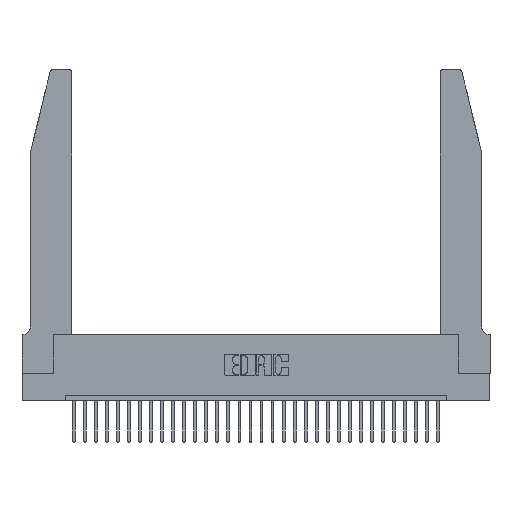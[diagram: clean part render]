
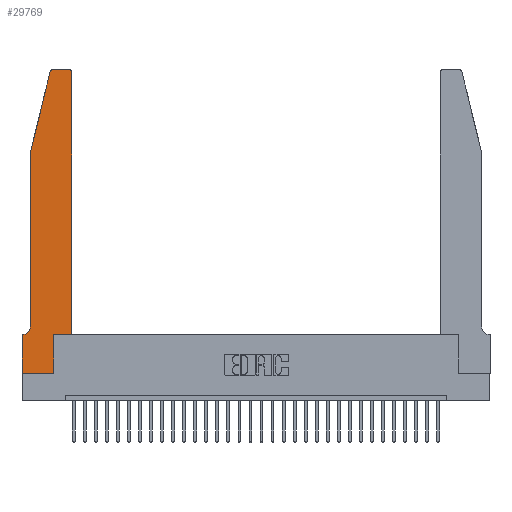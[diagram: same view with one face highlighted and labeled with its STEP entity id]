
A CAD part, top view. The second image highlights one B-rep face of the part: STEP entity #29769.
In plain terms, the highlighted planar face has unit normal (0, 0, 1).
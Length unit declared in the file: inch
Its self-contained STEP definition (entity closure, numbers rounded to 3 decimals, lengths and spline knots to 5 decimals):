
#386 = ORIENTED_EDGE ( 'NONE', *, *, #17840, .T. ) ;
#1127 = LINE ( 'NONE', #2753, #26141 ) ;
#1142 = EDGE_CURVE ( 'NONE', #30570, #8657, #6463, .T. ) ;
#1727 = ORIENTED_EDGE ( 'NONE', *, *, #22648, .T. ) ;
#2080 = ORIENTED_EDGE ( 'NONE', *, *, #17526, .T. ) ;
#2753 = CARTESIAN_POINT ( 'NONE',  ( 0., 0., 0.37 ) ) ;
#3370 = VECTOR ( 'NONE', #25159, 39.37008 ) ;
#3501 = EDGE_CURVE ( 'NONE', #26443, #23081, #20427, .T. ) ;
#3567 = CARTESIAN_POINT ( 'NONE',  ( 0.25487, 2.72718, 0.37 ) ) ;
#3782 = ORIENTED_EDGE ( 'NONE', *, *, #3501, .T. ) ;
#3824 = ORIENTED_EDGE ( 'NONE', *, *, #29797, .T. ) ;
#4398 = VERTEX_POINT ( 'NONE', #22264 ) ;
#4504 = VERTEX_POINT ( 'NONE', #17373 ) ;
#4585 = CARTESIAN_POINT ( 'NONE',  ( 0.284, 2.75, 0.37 ) ) ;
#4661 = DIRECTION ( 'NONE',  ( -1., 0., 0. ) ) ;
#4742 = VERTEX_POINT ( 'NONE', #24106 ) ;
#5469 = CARTESIAN_POINT ( 'NONE',  ( 0.0055, 0.42, 0.37 ) ) ;
#5599 = CARTESIAN_POINT ( 'NONE',  ( 0.4205, 2.72, 0.37 ) ) ;
#5793 = EDGE_CURVE ( 'NONE', #19160, #30570, #7446, .T. ) ;
#5992 = EDGE_CURVE ( 'NONE', #17692, #19160, #17774, .T. ) ;
#6463 = LINE ( 'NONE', #16593, #26981 ) ;
#6670 = CARTESIAN_POINT ( 'NONE',  ( 0.2865, 0.35, 0.37 ) ) ;
#6869 = CARTESIAN_POINT ( 'NONE',  ( 0.0755, 0.42, 0.37 ) ) ;
#7446 = LINE ( 'NONE', #19757, #18492 ) ;
#8516 = LINE ( 'NONE', #20334, #27184 ) ;
#8657 = VERTEX_POINT ( 'NONE', #20517 ) ;
#8892 = AXIS2_PLACEMENT_3D ( 'NONE', #27318, #10089, #29645 ) ;
#10089 = DIRECTION ( 'NONE',  ( 0., 0., 1. ) ) ;
#10143 = CARTESIAN_POINT ( 'NONE',  ( 0.2865, 0., 0.37 ) ) ;
#10771 = CARTESIAN_POINT ( 'NONE',  ( 0.0755, 2., 0.37 ) ) ;
#11291 = AXIS2_PLACEMENT_3D ( 'NONE', #27268, #14144, #31194 ) ;
#11407 = ORIENTED_EDGE ( 'NONE', *, *, #29382, .T. ) ;
#11547 = ORIENTED_EDGE ( 'NONE', *, *, #5992, .T. ) ;
#11615 = EDGE_CURVE ( 'NONE', #4504, #4398, #1127, .T. ) ;
#11762 = ORIENTED_EDGE ( 'NONE', *, *, #1142, .T. ) ;
#12613 = CARTESIAN_POINT ( 'NONE',  ( 0.2865, 0.35, 0.37 ) ) ;
#14035 = VECTOR ( 'NONE', #23655, 39.37008 ) ;
#14144 = DIRECTION ( 'NONE',  ( 0., 0., 1. ) ) ;
#14359 = LINE ( 'NONE', #14466, #19353 ) ;
#14362 = DIRECTION ( 'NONE',  ( 1., 0., 0. ) ) ;
#14466 = CARTESIAN_POINT ( 'NONE',  ( 0., 0., 0.37 ) ) ;
#14500 = DIRECTION ( 'NONE',  ( 1., 0., 0. ) ) ;
#14525 = PLANE ( 'NONE',  #8892 ) ;
#14882 = DIRECTION ( 'NONE',  ( 0., 0., 1. ) ) ;
#15059 = LINE ( 'NONE', #21736, #28769 ) ;
#15374 = ORIENTED_EDGE ( 'NONE', *, *, #21049, .T. ) ;
#16035 = VERTEX_POINT ( 'NONE', #20866 ) ;
#16593 = CARTESIAN_POINT ( 'NONE',  ( 0.4505, 0.35, 0.37 ) ) ;
#17159 = DIRECTION ( 'NONE',  ( 0., -1., 0. ) ) ;
#17358 = VECTOR ( 'NONE', #27774, 39.37008 ) ;
#17373 = CARTESIAN_POINT ( 'NONE',  ( 0., 0.35, 0.37 ) ) ;
#17526 = EDGE_CURVE ( 'NONE', #4398, #17692, #14359, .T. ) ;
#17539 = DIRECTION ( 'NONE',  ( -1., 0., 0. ) ) ;
#17692 = VERTEX_POINT ( 'NONE', #10143 ) ;
#17774 = LINE ( 'NONE', #12613, #3370 ) ;
#17840 = EDGE_CURVE ( 'NONE', #20067, #22050, #21230, .T. ) ;
#18263 = ORIENTED_EDGE ( 'NONE', *, *, #5793, .T. ) ;
#18492 = VECTOR ( 'NONE', #14500, 39.37008 ) ;
#19160 = VERTEX_POINT ( 'NONE', #6670 ) ;
#19353 = VECTOR ( 'NONE', #14362, 39.37008 ) ;
#19581 = CARTESIAN_POINT ( 'NONE',  ( 0.0755, 2., 0.37 ) ) ;
#19698 = DIRECTION ( 'NONE',  ( 1., 0., 0. ) ) ;
#19757 = CARTESIAN_POINT ( 'NONE',  ( 0.4505, 0.35, 0.37 ) ) ;
#20067 = VERTEX_POINT ( 'NONE', #19581 ) ;
#20119 = CIRCLE ( 'NONE', #25940, 0.03 ) ;
#20334 = CARTESIAN_POINT ( 'NONE',  ( 0.0755, 0.35, 0.37 ) ) ;
#20427 = CIRCLE ( 'NONE', #11291, 0.03 ) ;
#20517 = CARTESIAN_POINT ( 'NONE',  ( 0.4505, 2.72, 0.37 ) ) ;
#20866 = CARTESIAN_POINT ( 'NONE',  ( 0.4205, 2.75, 0.37 ) ) ;
#21049 = EDGE_CURVE ( 'NONE', #23081, #20067, #25824, .T. ) ;
#21230 = LINE ( 'NONE', #10771, #17358 ) ;
#21736 = CARTESIAN_POINT ( 'NONE',  ( 0.2605, 2.75, 0.37 ) ) ;
#22050 = VERTEX_POINT ( 'NONE', #6869 ) ;
#22264 = CARTESIAN_POINT ( 'NONE',  ( 0., 0., 0.37 ) ) ;
#22648 = EDGE_CURVE ( 'NONE', #16035, #26443, #15059, .T. ) ;
#22720 = ORIENTED_EDGE ( 'NONE', *, *, #27117, .T. ) ;
#23081 = VERTEX_POINT ( 'NONE', #3567 ) ;
#23343 = CARTESIAN_POINT ( 'NONE',  ( 0.0755, 2., 0.37 ) ) ;
#23655 = DIRECTION ( 'NONE',  ( -0.239, -0.971, 0. ) ) ;
#23716 = FACE_OUTER_BOUND ( 'NONE', #25717, .T. ) ;
#24106 = CARTESIAN_POINT ( 'NONE',  ( 0.0055, 0.35, 0.37 ) ) ;
#24869 = DIRECTION ( 'NONE',  ( 0., 0., -1. ) ) ;
#25159 = DIRECTION ( 'NONE',  ( 0., 1., 0. ) ) ;
#25361 = CARTESIAN_POINT ( 'NONE',  ( 0.4505, 0.35, 0.37 ) ) ;
#25717 = EDGE_LOOP ( 'NONE', ( #1727, #3782, #15374, #386, #3824, #11407, #30551, #2080, #11547, #18263, #11762, #22720 ) ) ;
#25824 = LINE ( 'NONE', #23343, #14035 ) ;
#25940 = AXIS2_PLACEMENT_3D ( 'NONE', #5599, #14882, #19698 ) ;
#26141 = VECTOR ( 'NONE', #17159, 39.37008 ) ;
#26443 = VERTEX_POINT ( 'NONE', #4585 ) ;
#26981 = VECTOR ( 'NONE', #31156, 39.37008 ) ;
#27117 = EDGE_CURVE ( 'NONE', #8657, #16035, #20119, .T. ) ;
#27184 = VECTOR ( 'NONE', #27647, 39.37008 ) ;
#27268 = CARTESIAN_POINT ( 'NONE',  ( 0.284, 2.72, 0.37 ) ) ;
#27318 = CARTESIAN_POINT ( 'NONE',  ( 0., 0.35, 0.37 ) ) ;
#27647 = DIRECTION ( 'NONE',  ( -1., 0., 0. ) ) ;
#27774 = DIRECTION ( 'NONE',  ( 0., -1., 0. ) ) ;
#28256 = CIRCLE ( 'NONE', #30279, 0.07 ) ;
#28769 = VECTOR ( 'NONE', #4661, 39.37008 ) ;
#29382 = EDGE_CURVE ( 'NONE', #4742, #4504, #8516, .T. ) ;
#29645 = DIRECTION ( 'NONE',  ( 1., 0., 0. ) ) ;
#29769 = ADVANCED_FACE ( 'NONE', ( #23716 ), #14525, .T. ) ;
#29797 = EDGE_CURVE ( 'NONE', #22050, #4742, #28256, .T. ) ;
#30279 = AXIS2_PLACEMENT_3D ( 'NONE', #5469, #24869, #17539 ) ;
#30551 = ORIENTED_EDGE ( 'NONE', *, *, #11615, .T. ) ;
#30570 = VERTEX_POINT ( 'NONE', #25361 ) ;
#31156 = DIRECTION ( 'NONE',  ( 0., 1., 0. ) ) ;
#31194 = DIRECTION ( 'NONE',  ( 1., 0., 0. ) ) ;
